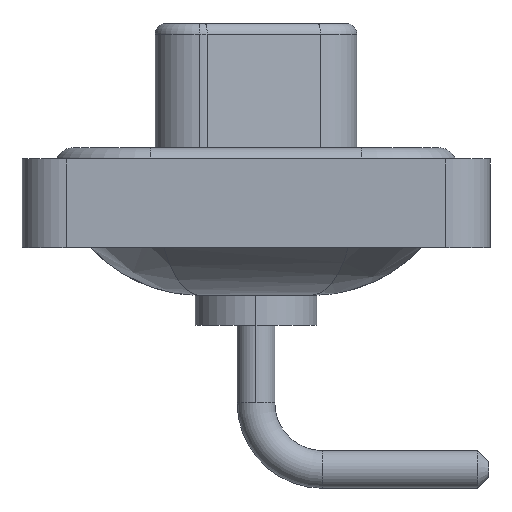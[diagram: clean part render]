
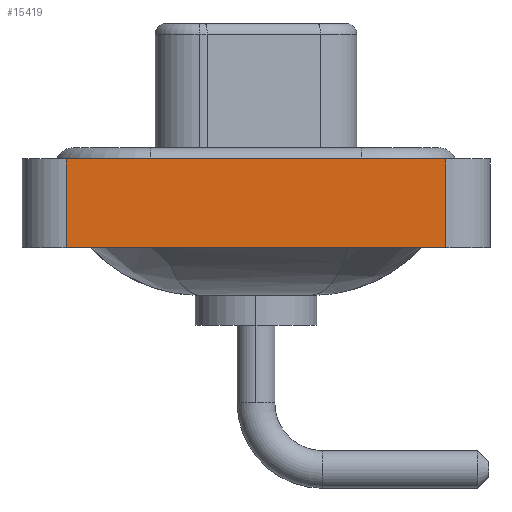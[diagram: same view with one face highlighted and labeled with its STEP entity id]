
A CAD part, left-side view. The second image highlights one B-rep face of the part: STEP entity #15419.
In plain terms, the highlighted planar face has unit normal (-1, 0, 0).
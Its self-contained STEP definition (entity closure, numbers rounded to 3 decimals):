
#82 = AXIS2_PLACEMENT_3D ( 'NONE', #3436, #3257, #2076 ) ;
#289 = CARTESIAN_POINT ( 'NONE',  ( -7.25, -8.55, -3.6 ) ) ;
#335 = CARTESIAN_POINT ( 'NONE',  ( -7.25, -8.55, -3.6 ) ) ;
#1548 = VERTEX_POINT ( 'NONE', #289 ) ;
#1660 = CARTESIAN_POINT ( 'NONE',  ( -7.25, -8.55, 0.4 ) ) ;
#1779 = EDGE_CURVE ( 'NONE', #4136, #15897, #4723, .T. ) ;
#2076 = DIRECTION ( 'NONE',  ( 0., 0., 1. ) ) ;
#2831 = ORIENTED_EDGE ( 'NONE', *, *, #17071, .T. ) ;
#3257 = DIRECTION ( 'NONE',  ( -1., 0., 0. ) ) ;
#3341 = FACE_OUTER_BOUND ( 'NONE', #15089, .T. ) ;
#3436 = CARTESIAN_POINT ( 'NONE',  ( -7.25, -8.55, -3.6 ) ) ;
#4136 = VERTEX_POINT ( 'NONE', #9649 ) ;
#4603 = CARTESIAN_POINT ( 'NONE',  ( -7.25, -8.55, -3.6 ) ) ;
#4680 = ORIENTED_EDGE ( 'NONE', *, *, #17507, .T. ) ;
#4685 = CARTESIAN_POINT ( 'NONE',  ( -7.25, 8.55, 0.4 ) ) ;
#4723 = LINE ( 'NONE', #12978, #9794 ) ;
#4787 = PLANE ( 'NONE',  #82 ) ;
#6167 = LINE ( 'NONE', #1660, #15826 ) ;
#7260 = DIRECTION ( 'NONE',  ( 0., -1., 0. ) ) ;
#7308 = VERTEX_POINT ( 'NONE', #9113 ) ;
#8960 = EDGE_CURVE ( 'NONE', #15897, #7308, #6167, .T. ) ;
#9044 = ORIENTED_EDGE ( 'NONE', *, *, #8960, .F. ) ;
#9113 = CARTESIAN_POINT ( 'NONE',  ( -7.25, -8.55, 0.4 ) ) ;
#9353 = ORIENTED_EDGE ( 'NONE', *, *, #1779, .F. ) ;
#9649 = CARTESIAN_POINT ( 'NONE',  ( -7.25, 8.55, -3.6 ) ) ;
#9794 = VECTOR ( 'NONE', #17326, 1000. ) ;
#10102 = DIRECTION ( 'NONE',  ( 0., 0., 1. ) ) ;
#10121 = DIRECTION ( 'NONE',  ( 0., -1., 0. ) ) ;
#12750 = LINE ( 'NONE', #335, #17266 ) ;
#12978 = CARTESIAN_POINT ( 'NONE',  ( -7.25, 8.55, -3.6 ) ) ;
#15089 = EDGE_LOOP ( 'NONE', ( #4680, #9044, #9353, #2831 ) ) ;
#15419 = ADVANCED_FACE ( 'NONE', ( #3341 ), #4787, .T. ) ;
#15521 = VECTOR ( 'NONE', #10121, 1000. ) ;
#15826 = VECTOR ( 'NONE', #7260, 1000. ) ;
#15897 = VERTEX_POINT ( 'NONE', #4685 ) ;
#17039 = LINE ( 'NONE', #4603, #15521 ) ;
#17071 = EDGE_CURVE ( 'NONE', #4136, #1548, #17039, .T. ) ;
#17266 = VECTOR ( 'NONE', #10102, 1000. ) ;
#17326 = DIRECTION ( 'NONE',  ( 0., 0., 1. ) ) ;
#17507 = EDGE_CURVE ( 'NONE', #1548, #7308, #12750, .T. ) ;
